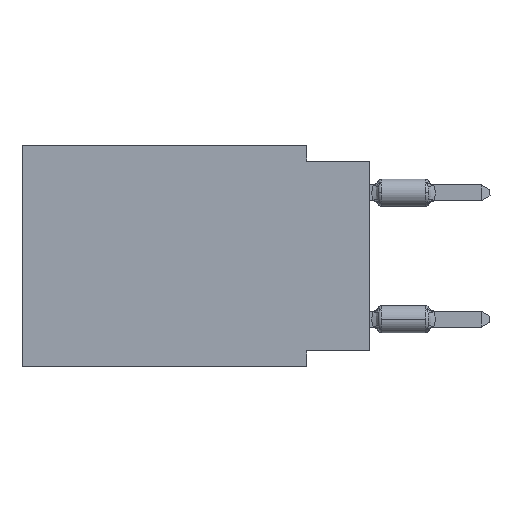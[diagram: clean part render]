
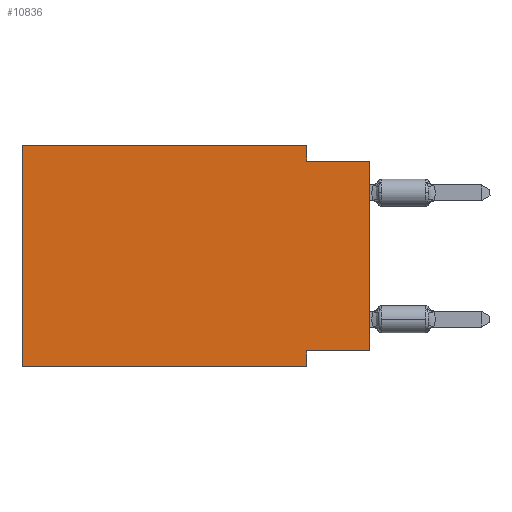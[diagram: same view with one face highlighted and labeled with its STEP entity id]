
A CAD part, left-side view. The second image highlights one B-rep face of the part: STEP entity #10836.
In plain terms, the highlighted planar face has unit normal (-1, 0, 0).
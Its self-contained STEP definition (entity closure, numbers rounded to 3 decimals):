
#292 = LINE ( 'NONE', #6548, #5678 ) ;
#295 = ORIENTED_EDGE ( 'NONE', *, *, #8437, .F. ) ;
#407 = VECTOR ( 'NONE', #2158, 1000. ) ;
#588 = ORIENTED_EDGE ( 'NONE', *, *, #12585, .T. ) ;
#1121 = LINE ( 'NONE', #11167, #1801 ) ;
#1330 = EDGE_CURVE ( 'NONE', #6158, #10092, #3778, .T. ) ;
#1519 = CARTESIAN_POINT ( 'NONE',  ( 0., 2.54, 0. ) ) ;
#1523 = AXIS2_PLACEMENT_3D ( 'NONE', #2477, #16227, #16312 ) ;
#1801 = VECTOR ( 'NONE', #12499, 1000. ) ;
#2087 = LINE ( 'NONE', #12330, #8923 ) ;
#2158 = DIRECTION ( 'NONE',  ( 0., 1., 0. ) ) ;
#2213 = ORIENTED_EDGE ( 'NONE', *, *, #12993, .F. ) ;
#2477 = CARTESIAN_POINT ( 'NONE',  ( 0., 13.97, 0. ) ) ;
#2812 = CARTESIAN_POINT ( 'NONE',  ( 0., 0., 0. ) ) ;
#2833 = EDGE_CURVE ( 'NONE', #9431, #11426, #1121, .T. ) ;
#3024 = VECTOR ( 'NONE', #4133, 1000. ) ;
#3514 = VERTEX_POINT ( 'NONE', #10528 ) ;
#3538 = ORIENTED_EDGE ( 'NONE', *, *, #14847, .T. ) ;
#3778 = LINE ( 'NONE', #12687, #10068 ) ;
#4079 = LINE ( 'NONE', #1519, #7917 ) ;
#4098 = ORIENTED_EDGE ( 'NONE', *, *, #10190, .F. ) ;
#4133 = DIRECTION ( 'NONE',  ( 0., 0., 1. ) ) ;
#4490 = VECTOR ( 'NONE', #5370, 1000. ) ;
#5370 = DIRECTION ( 'NONE',  ( 0., -1., 0. ) ) ;
#5477 = CARTESIAN_POINT ( 'NONE',  ( 0., 0., -0.635 ) ) ;
#5671 = CARTESIAN_POINT ( 'NONE',  ( 0., 13.97, -8.89 ) ) ;
#5678 = VECTOR ( 'NONE', #9077, 1000. ) ;
#5815 = EDGE_LOOP ( 'NONE', ( #3538, #2213, #4098, #295, #6582, #588, #14334, #13708 ) ) ;
#6158 = VERTEX_POINT ( 'NONE', #5671 ) ;
#6548 = CARTESIAN_POINT ( 'NONE',  ( 0., 13.97, -8.89 ) ) ;
#6582 = ORIENTED_EDGE ( 'NONE', *, *, #1330, .F. ) ;
#6990 = CARTESIAN_POINT ( 'NONE',  ( 0., 2.54, -8.255 ) ) ;
#7056 = CARTESIAN_POINT ( 'NONE',  ( 0., 2.54, 0. ) ) ;
#7431 = CARTESIAN_POINT ( 'NONE',  ( 0., 0., -8.255 ) ) ;
#7476 = DIRECTION ( 'NONE',  ( 0., 0., 1. ) ) ;
#7823 = CARTESIAN_POINT ( 'NONE',  ( 0., 13.97, 0. ) ) ;
#7917 = VECTOR ( 'NONE', #12911, 1000. ) ;
#8437 = EDGE_CURVE ( 'NONE', #10092, #12403, #10439, .T. ) ;
#8588 = PLANE ( 'NONE',  #1523 ) ;
#8923 = VECTOR ( 'NONE', #10806, 1000. ) ;
#9077 = DIRECTION ( 'NONE',  ( 0., -1., 0. ) ) ;
#9080 = CARTESIAN_POINT ( 'NONE',  ( 0., 2.54, -8.89 ) ) ;
#9170 = EDGE_CURVE ( 'NONE', #3514, #9431, #11302, .T. ) ;
#9247 = VERTEX_POINT ( 'NONE', #5477 ) ;
#9431 = VERTEX_POINT ( 'NONE', #6990 ) ;
#9565 = CARTESIAN_POINT ( 'NONE',  ( 0., 2.54, -0.635 ) ) ;
#9865 = VERTEX_POINT ( 'NONE', #9565 ) ;
#10068 = VECTOR ( 'NONE', #7476, 1000. ) ;
#10092 = VERTEX_POINT ( 'NONE', #10160 ) ;
#10160 = CARTESIAN_POINT ( 'NONE',  ( 0., 13.97, 0. ) ) ;
#10190 = EDGE_CURVE ( 'NONE', #12403, #9865, #4079, .T. ) ;
#10439 = LINE ( 'NONE', #7823, #4490 ) ;
#10528 = CARTESIAN_POINT ( 'NONE',  ( 0., 0., -8.255 ) ) ;
#10777 = FACE_OUTER_BOUND ( 'NONE', #5815, .T. ) ;
#10806 = DIRECTION ( 'NONE',  ( 0., -1., 0. ) ) ;
#10836 = ADVANCED_FACE ( 'NONE', ( #10777 ), #8588, .F. ) ;
#11167 = CARTESIAN_POINT ( 'NONE',  ( 0., 2.54, -8.89 ) ) ;
#11302 = LINE ( 'NONE', #7431, #407 ) ;
#11426 = VERTEX_POINT ( 'NONE', #9080 ) ;
#12330 = CARTESIAN_POINT ( 'NONE',  ( 0., 0., -0.635 ) ) ;
#12403 = VERTEX_POINT ( 'NONE', #7056 ) ;
#12499 = DIRECTION ( 'NONE',  ( 0., 0., -1. ) ) ;
#12585 = EDGE_CURVE ( 'NONE', #6158, #11426, #292, .T. ) ;
#12687 = CARTESIAN_POINT ( 'NONE',  ( 0., 13.97, 0. ) ) ;
#12888 = LINE ( 'NONE', #2812, #3024 ) ;
#12911 = DIRECTION ( 'NONE',  ( 0., 0., -1. ) ) ;
#12993 = EDGE_CURVE ( 'NONE', #9865, #9247, #2087, .T. ) ;
#13708 = ORIENTED_EDGE ( 'NONE', *, *, #9170, .F. ) ;
#14334 = ORIENTED_EDGE ( 'NONE', *, *, #2833, .F. ) ;
#14847 = EDGE_CURVE ( 'NONE', #3514, #9247, #12888, .T. ) ;
#16227 = DIRECTION ( 'NONE',  ( 1., 0., 0. ) ) ;
#16312 = DIRECTION ( 'NONE',  ( 0., 0., -1. ) ) ;
